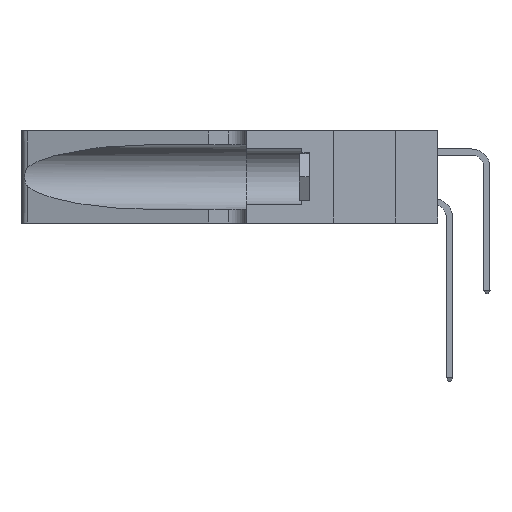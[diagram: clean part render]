
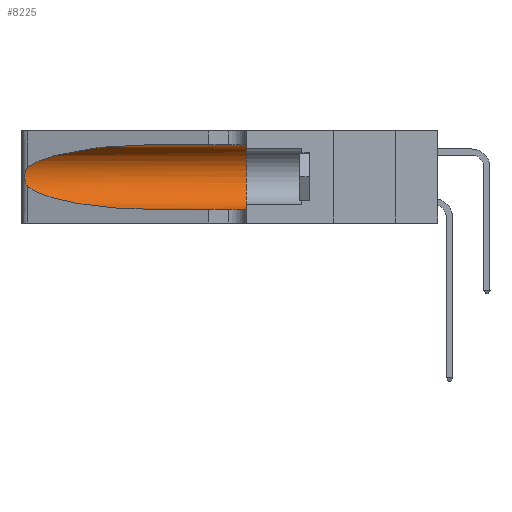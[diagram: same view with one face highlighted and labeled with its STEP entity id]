
A CAD part, left-side view. The second image highlights one B-rep face of the part: STEP entity #8225.
In plain terms, the highlighted cylindrical face has radius 3.308 mm (diameter 6.617 mm), a partial arc.
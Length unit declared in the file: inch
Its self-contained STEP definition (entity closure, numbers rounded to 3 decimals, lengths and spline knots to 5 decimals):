
#78 = VERTEX_POINT ( 'NONE', #15009 ) ;
#287 = AXIS2_PLACEMENT_3D ( 'NONE', #19336, #14332, #3251 ) ;
#1416 = EDGE_CURVE ( 'NONE', #11340, #10157, #18333, .T. ) ;
#1434 = CARTESIAN_POINT ( 'NONE',  ( 0.1305, 1.61858, 0.185 ) ) ;
#1698 = CARTESIAN_POINT ( 'NONE',  ( 0.25789, 1.23486, 0.15765 ) ) ;
#2870 = CARTESIAN_POINT ( 'NONE',  ( 0.25555, 1.22994, 0.2215 ) ) ;
#3243 = CARTESIAN_POINT ( 'NONE',  ( 0.18966, 0.96281, 0.31525 ) ) ;
#3251 = DIRECTION ( 'NONE',  ( 0., 0., 1. ) ) ;
#3366 = EDGE_CURVE ( 'NONE', #10157, #78, #9019, .T. ) ;
#4518 = CARTESIAN_POINT ( 'NONE',  ( 0.25854, 1.2359, 0.20912 ) ) ;
#4806 = CARTESIAN_POINT ( 'NONE',  ( 0.18966, 0.96281, 0.05475 ) ) ;
#5093 = CARTESIAN_POINT ( 'NONE',  ( 0.1305, 0.72297, 0.31525 ) ) ;
#6112 = CARTESIAN_POINT ( 'NONE',  ( 0.26018, 1.23835, 0.19895 ) ) ;
#6282 = CARTESIAN_POINT ( 'NONE',  ( 0.2373, 1.15595, 0.28018 ) ) ;
#6338 = CARTESIAN_POINT ( 'NONE',  ( 0.25487, 1.22718, 0.14631 ) ) ;
#7469 = CARTESIAN_POINT ( 'NONE',  ( 0.25487, 1.22718, 0.22369 ) ) ;
#7728 = CARTESIAN_POINT ( 'NONE',  ( 0.26075, 1.23896, 0.19203 ) ) ;
#7951 = AXIS2_PLACEMENT_3D ( 'NONE', #1434, #18380, #9015 ) ;
#8067 = CARTESIAN_POINT ( 'NONE',  ( 0.25555, 1.22993, 0.14849 ) ) ;
#8225 = ADVANCED_FACE ( 'NONE', ( #8381 ), #17615, .F. ) ;
#8234 =( BOUNDED_CURVE ( )  B_SPLINE_CURVE ( 3, ( #6338, #17582, #4806, #15899 ),
 .UNSPECIFIED., .F., .F. ) 
 B_SPLINE_CURVE_WITH_KNOTS ( ( 4, 4 ),
 ( 3.44316, 4.71239 ),
 .UNSPECIFIED. ) 
 CURVE ( )  GEOMETRIC_REPRESENTATION_ITEM ( )  RATIONAL_B_SPLINE_CURVE ( ( 1., 0.87, 0.87, 1. ) ) 
 REPRESENTATION_ITEM ( '' )  );
#8381 = FACE_OUTER_BOUND ( 'NONE', #19671, .T. ) ;
#9015 = DIRECTION ( 'NONE',  ( 0., 0., -1. ) ) ;
#9019 = CIRCLE ( 'NONE', #287, 0.13025 ) ;
#10157 = VERTEX_POINT ( 'NONE', #18906 ) ;
#11340 = VERTEX_POINT ( 'NONE', #5093 ) ;
#11441 = ORIENTED_EDGE ( 'NONE', *, *, #1416, .F. ) ;
#11691 = ORIENTED_EDGE ( 'NONE', *, *, #3366, .F. ) ;
#11695 = VERTEX_POINT ( 'NONE', #18896 ) ;
#12197 = CARTESIAN_POINT ( 'NONE',  ( 0.1305, 1.61858, 0.31525 ) ) ;
#12256 = EDGE_CURVE ( 'NONE', #12744, #78, #13972, .T. ) ;
#12509 = CARTESIAN_POINT ( 'NONE',  ( 0.25639, 1.23184, 0.21858 ) ) ;
#12744 = VERTEX_POINT ( 'NONE', #19110 ) ;
#12780 = CARTESIAN_POINT ( 'NONE',  ( 0.25639, 1.23186, 0.15144 ) ) ;
#12913 = CARTESIAN_POINT ( 'NONE',  ( 0.25487, 1.22718, 0.14631 ) ) ;
#13972 = LINE ( 'NONE', #14284, #18698 ) ;
#14141 = EDGE_CURVE ( 'NONE', #11340, #14497, #14757, .T. ) ;
#14261 = ORIENTED_EDGE ( 'NONE', *, *, #17369, .T. ) ;
#14284 = CARTESIAN_POINT ( 'NONE',  ( 0.1305, 1.61858, 0.05475 ) ) ;
#14332 = DIRECTION ( 'NONE',  ( 0., 1., 0. ) ) ;
#14497 = VERTEX_POINT ( 'NONE', #7469 ) ;
#14643 = ORIENTED_EDGE ( 'NONE', *, *, #18845, .T. ) ;
#14757 =( BOUNDED_CURVE ( )  B_SPLINE_CURVE ( 3, ( #15982, #3243, #6282, #18435 ),
 .UNSPECIFIED., .F., .F. ) 
 B_SPLINE_CURVE_WITH_KNOTS ( ( 4, 4 ),
 ( 1.5708, 2.84003 ),
 .UNSPECIFIED. ) 
 CURVE ( )  GEOMETRIC_REPRESENTATION_ITEM ( )  RATIONAL_B_SPLINE_CURVE ( ( 1., 0.87, 0.87, 1. ) ) 
 REPRESENTATION_ITEM ( '' )  );
#15009 = CARTESIAN_POINT ( 'NONE',  ( 0.1305, 0.35, 0.05475 ) ) ;
#15554 = CARTESIAN_POINT ( 'NONE',  ( 0.25487, 1.22718, 0.22369 ) ) ;
#15748 = CARTESIAN_POINT ( 'NONE',  ( 0.26017, 1.23833, 0.17102 ) ) ;
#15899 = CARTESIAN_POINT ( 'NONE',  ( 0.1305, 0.72297, 0.05475 ) ) ;
#15940 = DIRECTION ( 'NONE',  ( 0., -1., 0. ) ) ;
#15982 = CARTESIAN_POINT ( 'NONE',  ( 0.1305, 0.72297, 0.31525 ) ) ;
#16304 = VECTOR ( 'NONE', #16884, 39.37008 ) ;
#16884 = DIRECTION ( 'NONE',  ( 0., -1., 0. ) ) ;
#17348 = CARTESIAN_POINT ( 'NONE',  ( 0.25856, 1.23593, 0.16098 ) ) ;
#17369 = EDGE_CURVE ( 'NONE', #14497, #11695, #18479, .T. ) ;
#17582 = CARTESIAN_POINT ( 'NONE',  ( 0.2373, 1.15595, 0.08982 ) ) ;
#17615 = CYLINDRICAL_SURFACE ( 'NONE', #7951, 0.13025 ) ;
#18333 = LINE ( 'NONE', #12197, #16304 ) ;
#18380 = DIRECTION ( 'NONE',  ( 0., -1., 0. ) ) ;
#18435 = CARTESIAN_POINT ( 'NONE',  ( 0.25487, 1.22718, 0.22369 ) ) ;
#18479 = B_SPLINE_CURVE_WITH_KNOTS ( 'NONE', 3,
 ( #15554, #2870, #12509, #20458, #4518, #6112, #7728, #18897, #15748, #17348, #1698, #12780, #8067, #12913 ),
 .UNSPECIFIED., .F., .F.,
 ( 4, 2, 2, 2, 2, 2, 4 ),
 ( 0., 0.00027, 0.00053, 0.00107, 0.0016, 0.00187, 0.00214 ),
 .UNSPECIFIED. ) ;
#18698 = VECTOR ( 'NONE', #15940, 39.37008 ) ;
#18845 = EDGE_CURVE ( 'NONE', #11695, #12744, #8234, .T. ) ;
#18896 = CARTESIAN_POINT ( 'NONE',  ( 0.25487, 1.22718, 0.14631 ) ) ;
#18897 = CARTESIAN_POINT ( 'NONE',  ( 0.26075, 1.23896, 0.178 ) ) ;
#18906 = CARTESIAN_POINT ( 'NONE',  ( 0.1305, 0.35, 0.31525 ) ) ;
#19110 = CARTESIAN_POINT ( 'NONE',  ( 0.1305, 0.72297, 0.05475 ) ) ;
#19336 = CARTESIAN_POINT ( 'NONE',  ( 0.1305, 0.35, 0.185 ) ) ;
#19671 = EDGE_LOOP ( 'NONE', ( #20572, #14261, #14643, #20169, #11691, #11441 ) ) ;
#20169 = ORIENTED_EDGE ( 'NONE', *, *, #12256, .T. ) ;
#20458 = CARTESIAN_POINT ( 'NONE',  ( 0.25787, 1.23484, 0.2124 ) ) ;
#20572 = ORIENTED_EDGE ( 'NONE', *, *, #14141, .T. ) ;
